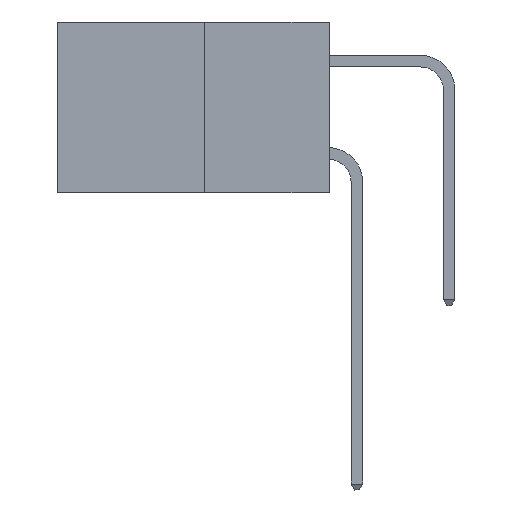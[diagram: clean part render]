
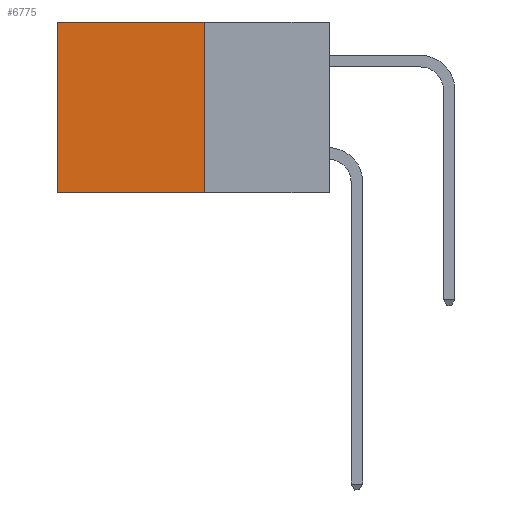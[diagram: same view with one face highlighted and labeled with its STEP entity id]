
A CAD part, left-side view. The second image highlights one B-rep face of the part: STEP entity #6775.
In plain terms, the highlighted planar face has unit normal (-1, 0, 0).
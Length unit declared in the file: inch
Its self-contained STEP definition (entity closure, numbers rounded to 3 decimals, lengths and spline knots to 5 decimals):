
#22 = EDGE_CURVE ( 'NONE', #750, #15310, #17971, .T. ) ;
#750 = VERTEX_POINT ( 'NONE', #11053 ) ;
#1300 = ORIENTED_EDGE ( 'NONE', *, *, #25493, .F. ) ;
#1557 = ORIENTED_EDGE ( 'NONE', *, *, #16803, .F. ) ;
#1565 = EDGE_CURVE ( 'NONE', #11201, #750, #26101, .T. ) ;
#1843 = CARTESIAN_POINT ( 'NONE',  ( 0.277, 0.59, -0.37 ) ) ;
#3180 = EDGE_LOOP ( 'NONE', ( #24828, #1300, #1557, #29800 ) ) ;
#3247 = DIRECTION ( 'NONE',  ( 0., 0., -1. ) ) ;
#4098 = VECTOR ( 'NONE', #14136, 39.37008 ) ;
#6775 = ADVANCED_FACE ( 'NONE', ( #7798 ), #25670, .F. ) ;
#7481 = VECTOR ( 'NONE', #20064, 39.37008 ) ;
#7798 = FACE_OUTER_BOUND ( 'NONE', #3180, .T. ) ;
#10271 = CARTESIAN_POINT ( 'NONE',  ( 0.277, 0.27, 0. ) ) ;
#10639 = VECTOR ( 'NONE', #3247, 39.37008 ) ;
#11053 = CARTESIAN_POINT ( 'NONE',  ( 0.277, 0.59, 0. ) ) ;
#11201 = VERTEX_POINT ( 'NONE', #15173 ) ;
#11940 = CARTESIAN_POINT ( 'NONE',  ( 0.277, 0.27, -0.37 ) ) ;
#12707 = CARTESIAN_POINT ( 'NONE',  ( 0.277, 0.27, -0.37 ) ) ;
#14136 = DIRECTION ( 'NONE',  ( 0., 1., 0. ) ) ;
#15173 = CARTESIAN_POINT ( 'NONE',  ( 0.277, 0.27, 0. ) ) ;
#15310 = VERTEX_POINT ( 'NONE', #30255 ) ;
#15465 = DIRECTION ( 'NONE',  ( 0., 1., 0. ) ) ;
#16803 = EDGE_CURVE ( 'NONE', #11201, #28021, #22144, .T. ) ;
#17282 = CARTESIAN_POINT ( 'NONE',  ( 0.277, 0.27, -0.37 ) ) ;
#17460 = DIRECTION ( 'NONE',  ( 0., 0., -1. ) ) ;
#17883 = VECTOR ( 'NONE', #15465, 39.37008 ) ;
#17971 = LINE ( 'NONE', #1843, #10639 ) ;
#19601 = LINE ( 'NONE', #12707, #17883 ) ;
#20064 = DIRECTION ( 'NONE',  ( 0., 0., -1. ) ) ;
#20998 = AXIS2_PLACEMENT_3D ( 'NONE', #11940, #33927, #17460 ) ;
#22144 = LINE ( 'NONE', #17282, #7481 ) ;
#24828 = ORIENTED_EDGE ( 'NONE', *, *, #22, .T. ) ;
#25493 = EDGE_CURVE ( 'NONE', #28021, #15310, #19601, .T. ) ;
#25670 = PLANE ( 'NONE',  #20998 ) ;
#26101 = LINE ( 'NONE', #10271, #4098 ) ;
#27526 = CARTESIAN_POINT ( 'NONE',  ( 0.277, 0.27, -0.37 ) ) ;
#28021 = VERTEX_POINT ( 'NONE', #27526 ) ;
#29800 = ORIENTED_EDGE ( 'NONE', *, *, #1565, .T. ) ;
#30255 = CARTESIAN_POINT ( 'NONE',  ( 0.277, 0.59, -0.37 ) ) ;
#33927 = DIRECTION ( 'NONE',  ( 1., 0., 0. ) ) ;
